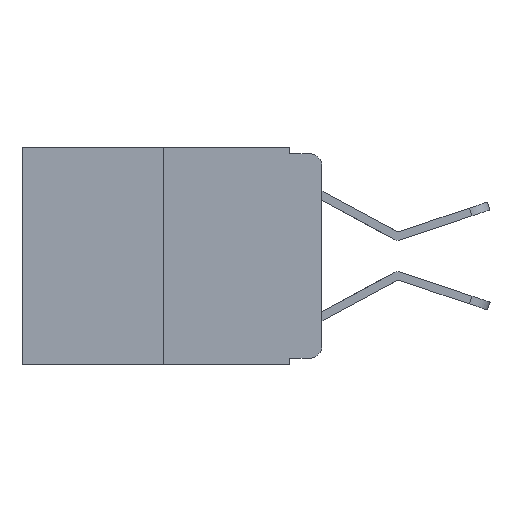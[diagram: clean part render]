
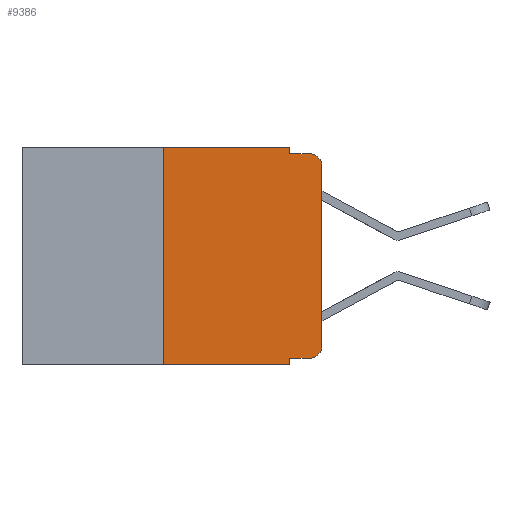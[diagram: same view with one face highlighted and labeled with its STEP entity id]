
A CAD part, left-side view. The second image highlights one B-rep face of the part: STEP entity #9386.
In plain terms, the highlighted planar face has unit normal (-1, 0, 0).
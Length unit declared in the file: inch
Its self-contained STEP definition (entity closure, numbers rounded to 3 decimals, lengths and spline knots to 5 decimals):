
#166 = DIRECTION ( 'NONE',  ( 0., -1., 0. ) ) ;
#332 = DIRECTION ( 'NONE',  ( 0., 0., 1. ) ) ;
#587 = EDGE_CURVE ( 'NONE', #8425, #7650, #10191, .T. ) ;
#618 = VERTEX_POINT ( 'NONE', #3724 ) ;
#901 = FACE_OUTER_BOUND ( 'NONE', #4732, .T. ) ;
#976 = DIRECTION ( 'NONE',  ( -1., 0., 0. ) ) ;
#1526 = EDGE_CURVE ( 'NONE', #3636, #8425, #12541, .T. ) ;
#1659 = VECTOR ( 'NONE', #11471, 39.37008 ) ;
#1709 = CARTESIAN_POINT ( 'NONE',  ( 0., 0.02, -0.03 ) ) ;
#2290 = CARTESIAN_POINT ( 'NONE',  ( 0., 0.473, 0. ) ) ;
#2415 = EDGE_CURVE ( 'NONE', #618, #13040, #6199, .T. ) ;
#2663 = CARTESIAN_POINT ( 'NONE',  ( 0., 0.051, 0. ) ) ;
#2697 = DIRECTION ( 'NONE',  ( 0., 0., -1. ) ) ;
#2722 = VERTEX_POINT ( 'NONE', #3515 ) ;
#2733 = AXIS2_PLACEMENT_3D ( 'NONE', #1709, #3861, #2697 ) ;
#2858 = EDGE_CURVE ( 'NONE', #13040, #3945, #9533, .T. ) ;
#3162 = DIRECTION ( 'NONE',  ( 1., 0., 0. ) ) ;
#3208 = CARTESIAN_POINT ( 'NONE',  ( 0., 0.473, 0. ) ) ;
#3271 = EDGE_CURVE ( 'NONE', #3945, #7650, #13472, .T. ) ;
#3448 = ORIENTED_EDGE ( 'NONE', *, *, #2415, .F. ) ;
#3474 = ORIENTED_EDGE ( 'NONE', *, *, #11333, .F. ) ;
#3479 = CARTESIAN_POINT ( 'NONE',  ( 0., 0.051, -0.333 ) ) ;
#3515 = CARTESIAN_POINT ( 'NONE',  ( 0., 0.25, -0.343 ) ) ;
#3636 = VERTEX_POINT ( 'NONE', #8051 ) ;
#3724 = CARTESIAN_POINT ( 'NONE',  ( 0., 0.25, 0. ) ) ;
#3741 = DIRECTION ( 'NONE',  ( 0., 0., -1. ) ) ;
#3858 = VECTOR ( 'NONE', #3741, 39.37008 ) ;
#3861 = DIRECTION ( 'NONE',  ( -1., 0., 0. ) ) ;
#3945 = VERTEX_POINT ( 'NONE', #5448 ) ;
#3968 = DIRECTION ( 'NONE',  ( 0., -1., 0. ) ) ;
#4136 = DIRECTION ( 'NONE',  ( 0., 0., -1. ) ) ;
#4194 = VECTOR ( 'NONE', #332, 39.37008 ) ;
#4562 = VERTEX_POINT ( 'NONE', #3479 ) ;
#4732 = EDGE_LOOP ( 'NONE', ( #6873, #6841, #8932, #8301, #3448, #3474, #10765, #10976, #10194, #5873 ) ) ;
#4937 = CARTESIAN_POINT ( 'NONE',  ( 0., 0., -0.03 ) ) ;
#5111 = LINE ( 'NONE', #6248, #9775 ) ;
#5203 = CARTESIAN_POINT ( 'NONE',  ( 0., 0.051, -0.333 ) ) ;
#5448 = CARTESIAN_POINT ( 'NONE',  ( 0., 0.051, -0.01 ) ) ;
#5738 = CARTESIAN_POINT ( 'NONE',  ( 0., 0.02, -0.01 ) ) ;
#5873 = ORIENTED_EDGE ( 'NONE', *, *, #9887, .T. ) ;
#6004 = LINE ( 'NONE', #13268, #4194 ) ;
#6199 = LINE ( 'NONE', #2290, #12359 ) ;
#6248 = CARTESIAN_POINT ( 'NONE',  ( 0., 0.051, 0. ) ) ;
#6470 = CARTESIAN_POINT ( 'NONE',  ( 0., 0.02, -0.333 ) ) ;
#6841 = ORIENTED_EDGE ( 'NONE', *, *, #587, .T. ) ;
#6873 = ORIENTED_EDGE ( 'NONE', *, *, #1526, .T. ) ;
#7186 = CARTESIAN_POINT ( 'NONE',  ( 0., 0.02, -0.313 ) ) ;
#7312 = CARTESIAN_POINT ( 'NONE',  ( 0., 0.051, -0.01 ) ) ;
#7388 = CIRCLE ( 'NONE', #12791, 0.02 ) ;
#7417 = EDGE_CURVE ( 'NONE', #4562, #8883, #10734, .T. ) ;
#7650 = VERTEX_POINT ( 'NONE', #5738 ) ;
#7936 = EDGE_CURVE ( 'NONE', #4562, #12069, #5111, .T. ) ;
#8051 = CARTESIAN_POINT ( 'NONE',  ( 0., 0., -0.313 ) ) ;
#8101 = CARTESIAN_POINT ( 'NONE',  ( 0., 0.473, -0.343 ) ) ;
#8238 = DIRECTION ( 'NONE',  ( 0., 0., -1. ) ) ;
#8301 = ORIENTED_EDGE ( 'NONE', *, *, #2858, .F. ) ;
#8377 = DIRECTION ( 'NONE',  ( 0., -1., 0. ) ) ;
#8425 = VERTEX_POINT ( 'NONE', #4937 ) ;
#8451 = CARTESIAN_POINT ( 'NONE',  ( 0., 0., 0. ) ) ;
#8883 = VERTEX_POINT ( 'NONE', #6470 ) ;
#8932 = ORIENTED_EDGE ( 'NONE', *, *, #3271, .F. ) ;
#9177 = VECTOR ( 'NONE', #8377, 39.37008 ) ;
#9386 = ADVANCED_FACE ( 'NONE', ( #901 ), #10501, .F. ) ;
#9533 = LINE ( 'NONE', #2663, #3858 ) ;
#9535 = DIRECTION ( 'NONE',  ( 0., 0., 1. ) ) ;
#9725 = CARTESIAN_POINT ( 'NONE',  ( 0., 0.051, 0. ) ) ;
#9775 = VECTOR ( 'NONE', #10445, 39.37008 ) ;
#9887 = EDGE_CURVE ( 'NONE', #8883, #3636, #7388, .T. ) ;
#10122 = CARTESIAN_POINT ( 'NONE',  ( 0., 0.051, -0.343 ) ) ;
#10191 = CIRCLE ( 'NONE', #2733, 0.02 ) ;
#10194 = ORIENTED_EDGE ( 'NONE', *, *, #7417, .T. ) ;
#10225 = VECTOR ( 'NONE', #3968, 39.37008 ) ;
#10320 = LINE ( 'NONE', #8101, #1659 ) ;
#10445 = DIRECTION ( 'NONE',  ( 0., 0., -1. ) ) ;
#10501 = PLANE ( 'NONE',  #11824 ) ;
#10734 = LINE ( 'NONE', #5203, #10225 ) ;
#10765 = ORIENTED_EDGE ( 'NONE', *, *, #12122, .T. ) ;
#10976 = ORIENTED_EDGE ( 'NONE', *, *, #7936, .F. ) ;
#11333 = EDGE_CURVE ( 'NONE', #2722, #618, #6004, .T. ) ;
#11471 = DIRECTION ( 'NONE',  ( 0., -1., 0. ) ) ;
#11824 = AXIS2_PLACEMENT_3D ( 'NONE', #3208, #3162, #4136 ) ;
#12069 = VERTEX_POINT ( 'NONE', #10122 ) ;
#12122 = EDGE_CURVE ( 'NONE', #2722, #12069, #10320, .T. ) ;
#12359 = VECTOR ( 'NONE', #166, 39.37008 ) ;
#12541 = LINE ( 'NONE', #8451, #13182 ) ;
#12791 = AXIS2_PLACEMENT_3D ( 'NONE', #7186, #976, #8238 ) ;
#13040 = VERTEX_POINT ( 'NONE', #9725 ) ;
#13182 = VECTOR ( 'NONE', #9535, 39.37008 ) ;
#13268 = CARTESIAN_POINT ( 'NONE',  ( 0., 0.25, 0. ) ) ;
#13472 = LINE ( 'NONE', #7312, #9177 ) ;
